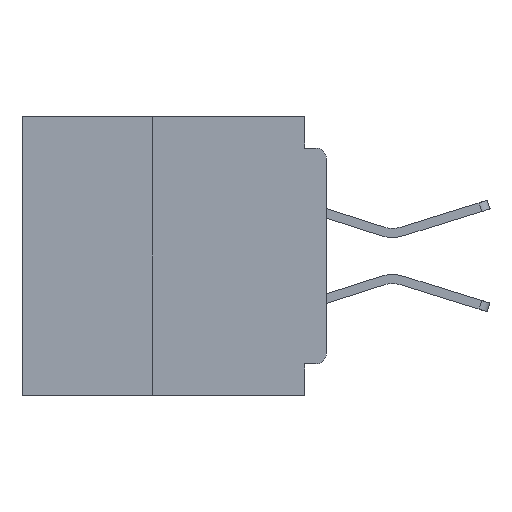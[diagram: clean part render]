
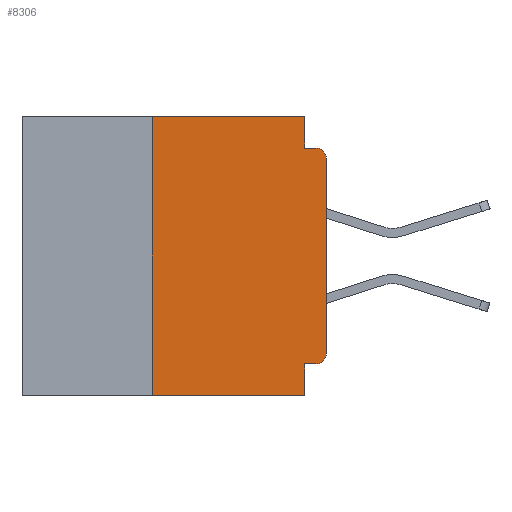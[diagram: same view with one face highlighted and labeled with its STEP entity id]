
A CAD part, left-side view. The second image highlights one B-rep face of the part: STEP entity #8306.
In plain terms, the highlighted planar face has unit normal (-1, 0, 0).
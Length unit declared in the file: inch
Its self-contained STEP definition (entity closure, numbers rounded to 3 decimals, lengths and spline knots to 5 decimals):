
#132 = LINE ( 'NONE', #14594, #37630 ) ;
#195 = ORIENTED_EDGE ( 'NONE', *, *, #29473, .F. ) ;
#445 = VECTOR ( 'NONE', #12043, 39.37008 ) ;
#898 = VERTEX_POINT ( 'NONE', #15656 ) ;
#981 = CARTESIAN_POINT ( 'NONE',  ( 0., 0.031, 0. ) ) ;
#1534 = VECTOR ( 'NONE', #24271, 39.37008 ) ;
#1748 = CARTESIAN_POINT ( 'NONE',  ( 0., 0.437, 0. ) ) ;
#2874 = EDGE_CURVE ( 'NONE', #9554, #8552, #40170, .T. ) ;
#3128 = CIRCLE ( 'NONE', #35307, 0.015 ) ;
#3927 = EDGE_CURVE ( 'NONE', #14055, #8552, #3128, .T. ) ;
#4464 = CARTESIAN_POINT ( 'NONE',  ( 0., 0., -0.34 ) ) ;
#5087 = CARTESIAN_POINT ( 'NONE',  ( 0., 0.437, 0. ) ) ;
#5267 = EDGE_CURVE ( 'NONE', #10033, #9554, #14962, .T. ) ;
#5744 = ORIENTED_EDGE ( 'NONE', *, *, #3927, .T. ) ;
#7525 = DIRECTION ( 'NONE',  ( 0., 1., 0. ) ) ;
#8306 = ADVANCED_FACE ( 'NONE', ( #44755 ), #26824, .F. ) ;
#8552 = VERTEX_POINT ( 'NONE', #35590 ) ;
#8748 = DIRECTION ( 'NONE',  ( 1., 0., 0. ) ) ;
#9252 = VECTOR ( 'NONE', #7525, 39.37008 ) ;
#9554 = VERTEX_POINT ( 'NONE', #23356 ) ;
#9819 = ORIENTED_EDGE ( 'NONE', *, *, #23468, .F. ) ;
#10033 = VERTEX_POINT ( 'NONE', #981 ) ;
#10123 = LINE ( 'NONE', #19171, #445 ) ;
#10458 = ORIENTED_EDGE ( 'NONE', *, *, #28790, .T. ) ;
#10861 = ORIENTED_EDGE ( 'NONE', *, *, #44810, .T. ) ;
#11234 = CARTESIAN_POINT ( 'NONE',  ( 0., 0.015, -0.34 ) ) ;
#11490 = EDGE_CURVE ( 'NONE', #898, #41936, #14757, .T. ) ;
#12043 = DIRECTION ( 'NONE',  ( 0., 0., -1. ) ) ;
#12717 = ORIENTED_EDGE ( 'NONE', *, *, #44740, .T. ) ;
#14055 = VERTEX_POINT ( 'NONE', #23850 ) ;
#14594 = CARTESIAN_POINT ( 'NONE',  ( 0., 0.437, -0.4 ) ) ;
#14757 = LINE ( 'NONE', #26705, #22042 ) ;
#14905 = DIRECTION ( 'NONE',  ( 0., 0., -1. ) ) ;
#14962 = LINE ( 'NONE', #40220, #31958 ) ;
#15547 = VECTOR ( 'NONE', #29590, 39.37008 ) ;
#15656 = CARTESIAN_POINT ( 'NONE',  ( 0., 0.25, -0.4 ) ) ;
#16111 = ORIENTED_EDGE ( 'NONE', *, *, #18647, .F. ) ;
#17540 = AXIS2_PLACEMENT_3D ( 'NONE', #5087, #8748, #34157 ) ;
#18647 = EDGE_CURVE ( 'NONE', #44603, #31760, #10123, .T. ) ;
#19171 = CARTESIAN_POINT ( 'NONE',  ( 0., 0.031, -0.4 ) ) ;
#19209 = CARTESIAN_POINT ( 'NONE',  ( 0., 0.015, -0.355 ) ) ;
#20723 = EDGE_LOOP ( 'NONE', ( #10861, #5744, #44452, #28527, #9819, #22837, #12717, #16111, #195, #10458 ) ) ;
#22042 = VECTOR ( 'NONE', #30365, 39.37008 ) ;
#22837 = ORIENTED_EDGE ( 'NONE', *, *, #11490, .F. ) ;
#23356 = CARTESIAN_POINT ( 'NONE',  ( 0., 0.031, -0.045 ) ) ;
#23468 = EDGE_CURVE ( 'NONE', #41936, #10033, #38960, .T. ) ;
#23632 = CARTESIAN_POINT ( 'NONE',  ( 0., 0., -0.045 ) ) ;
#23850 = CARTESIAN_POINT ( 'NONE',  ( 0., 0., -0.06 ) ) ;
#24271 = DIRECTION ( 'NONE',  ( 0., -1., 0. ) ) ;
#25671 = LINE ( 'NONE', #25949, #15547 ) ;
#25949 = CARTESIAN_POINT ( 'NONE',  ( 0., 0., 0. ) ) ;
#26705 = CARTESIAN_POINT ( 'NONE',  ( 0., 0.25, -0.4 ) ) ;
#26824 = PLANE ( 'NONE',  #17540 ) ;
#28527 = ORIENTED_EDGE ( 'NONE', *, *, #5267, .F. ) ;
#28561 = LINE ( 'NONE', #29234, #9252 ) ;
#28790 = EDGE_CURVE ( 'NONE', #35682, #43507, #30316, .T. ) ;
#29234 = CARTESIAN_POINT ( 'NONE',  ( 0., 0., -0.355 ) ) ;
#29473 = EDGE_CURVE ( 'NONE', #35682, #44603, #28561, .T. ) ;
#29590 = DIRECTION ( 'NONE',  ( 0., 0., 1. ) ) ;
#30316 = CIRCLE ( 'NONE', #42239, 0.015 ) ;
#30365 = DIRECTION ( 'NONE',  ( 0., 0., 1. ) ) ;
#31760 = VERTEX_POINT ( 'NONE', #43310 ) ;
#31958 = VECTOR ( 'NONE', #43731, 39.37008 ) ;
#31971 = CARTESIAN_POINT ( 'NONE',  ( 0., 0.25, 0. ) ) ;
#32638 = DIRECTION ( 'NONE',  ( 0., -1., 0. ) ) ;
#34157 = DIRECTION ( 'NONE',  ( 0., 0., -1. ) ) ;
#34467 = DIRECTION ( 'NONE',  ( 0., -1., 0. ) ) ;
#35307 = AXIS2_PLACEMENT_3D ( 'NONE', #46148, #45980, #45936 ) ;
#35590 = CARTESIAN_POINT ( 'NONE',  ( 0., 0.015, -0.045 ) ) ;
#35682 = VERTEX_POINT ( 'NONE', #19209 ) ;
#36621 = DIRECTION ( 'NONE',  ( -1., 0., 0. ) ) ;
#37630 = VECTOR ( 'NONE', #32638, 39.37008 ) ;
#37823 = VECTOR ( 'NONE', #34467, 39.37008 ) ;
#38960 = LINE ( 'NONE', #1748, #37823 ) ;
#39171 = CARTESIAN_POINT ( 'NONE',  ( 0., 0.031, -0.355 ) ) ;
#40170 = LINE ( 'NONE', #23632, #1534 ) ;
#40220 = CARTESIAN_POINT ( 'NONE',  ( 0., 0.031, 0. ) ) ;
#41936 = VERTEX_POINT ( 'NONE', #31971 ) ;
#42239 = AXIS2_PLACEMENT_3D ( 'NONE', #11234, #36621, #14905 ) ;
#43310 = CARTESIAN_POINT ( 'NONE',  ( 0., 0.031, -0.4 ) ) ;
#43507 = VERTEX_POINT ( 'NONE', #4464 ) ;
#43731 = DIRECTION ( 'NONE',  ( 0., 0., -1. ) ) ;
#44452 = ORIENTED_EDGE ( 'NONE', *, *, #2874, .F. ) ;
#44603 = VERTEX_POINT ( 'NONE', #39171 ) ;
#44740 = EDGE_CURVE ( 'NONE', #898, #31760, #132, .T. ) ;
#44755 = FACE_OUTER_BOUND ( 'NONE', #20723, .T. ) ;
#44810 = EDGE_CURVE ( 'NONE', #43507, #14055, #25671, .T. ) ;
#45936 = DIRECTION ( 'NONE',  ( 0., 0., -1. ) ) ;
#45980 = DIRECTION ( 'NONE',  ( -1., 0., 0. ) ) ;
#46148 = CARTESIAN_POINT ( 'NONE',  ( 0., 0.015, -0.06 ) ) ;
